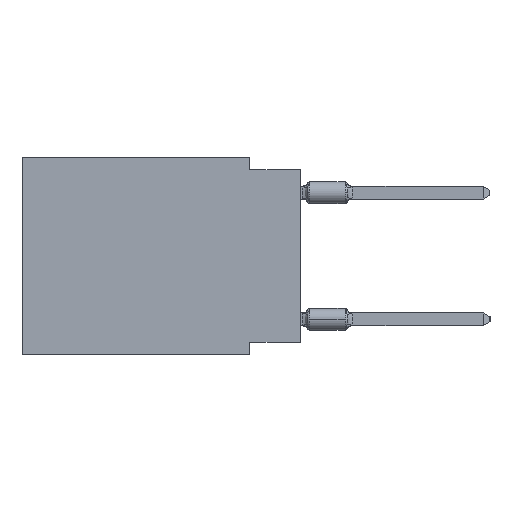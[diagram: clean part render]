
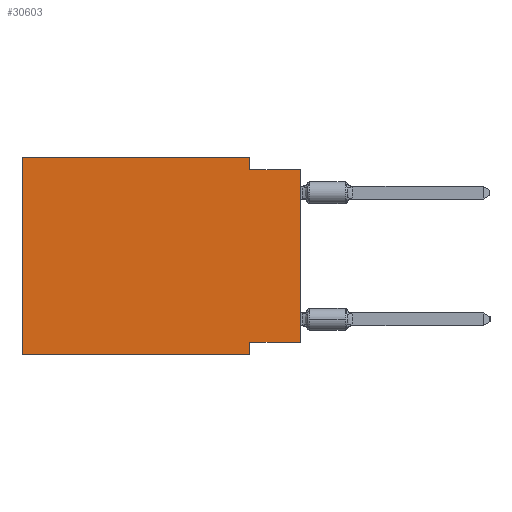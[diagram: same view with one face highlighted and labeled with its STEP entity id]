
A CAD part, left-side view. The second image highlights one B-rep face of the part: STEP entity #30603.
In plain terms, the highlighted planar face has unit normal (-1, 0, 0).
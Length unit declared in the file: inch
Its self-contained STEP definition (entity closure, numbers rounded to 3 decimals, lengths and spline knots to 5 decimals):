
#1316 = CARTESIAN_POINT ( 'NONE',  ( 0., 0.1, 0. ) ) ;
#1933 = EDGE_CURVE ( 'NONE', #29544, #7991, #47977, .T. ) ;
#4544 = DIRECTION ( 'NONE',  ( 0., 1., 0. ) ) ;
#4840 = FACE_OUTER_BOUND ( 'NONE', #44132, .T. ) ;
#5607 = VERTEX_POINT ( 'NONE', #27219 ) ;
#6581 = CARTESIAN_POINT ( 'NONE',  ( 0., 0.1, -0.365 ) ) ;
#7967 = CARTESIAN_POINT ( 'NONE',  ( 0., 0., -0.365 ) ) ;
#7991 = VERTEX_POINT ( 'NONE', #42795 ) ;
#8551 = ORIENTED_EDGE ( 'NONE', *, *, #11767, .F. ) ;
#9756 = LINE ( 'NONE', #56071, #59518 ) ;
#10496 = VERTEX_POINT ( 'NONE', #6581 ) ;
#10567 = LINE ( 'NONE', #16376, #41901 ) ;
#11022 = VERTEX_POINT ( 'NONE', #48261 ) ;
#11767 = EDGE_CURVE ( 'NONE', #47451, #29544, #20997, .T. ) ;
#12686 = CARTESIAN_POINT ( 'NONE',  ( 0., 0.55, 0. ) ) ;
#12874 = ORIENTED_EDGE ( 'NONE', *, *, #43140, .F. ) ;
#14507 = VECTOR ( 'NONE', #36011, 39.37008 ) ;
#14711 = EDGE_CURVE ( 'NONE', #5607, #11022, #17626, .T. ) ;
#16376 = CARTESIAN_POINT ( 'NONE',  ( 0., 0., -0.025 ) ) ;
#16868 = CARTESIAN_POINT ( 'NONE',  ( 0., 0.55, -0.39 ) ) ;
#17626 = LINE ( 'NONE', #45534, #57797 ) ;
#18525 = VECTOR ( 'NONE', #27995, 39.37008 ) ;
#20997 = LINE ( 'NONE', #12686, #14507 ) ;
#23380 = LINE ( 'NONE', #56791, #18525 ) ;
#23572 = DIRECTION ( 'NONE',  ( 1., 0., 0. ) ) ;
#24297 = ORIENTED_EDGE ( 'NONE', *, *, #55354, .F. ) ;
#25605 = ORIENTED_EDGE ( 'NONE', *, *, #1933, .F. ) ;
#26970 = DIRECTION ( 'NONE',  ( 0., -1., 0. ) ) ;
#27219 = CARTESIAN_POINT ( 'NONE',  ( 0., 0., -0.365 ) ) ;
#27995 = DIRECTION ( 'NONE',  ( 0., 0., 1. ) ) ;
#28317 = EDGE_CURVE ( 'NONE', #7991, #11022, #10567, .T. ) ;
#29544 = VERTEX_POINT ( 'NONE', #54392 ) ;
#29685 = CARTESIAN_POINT ( 'NONE',  ( 0., 0.55, 0. ) ) ;
#30205 = AXIS2_PLACEMENT_3D ( 'NONE', #37084, #23572, #37987 ) ;
#30603 = ADVANCED_FACE ( 'NONE', ( #4840 ), #37394, .F. ) ;
#30870 = ORIENTED_EDGE ( 'NONE', *, *, #40388, .F. ) ;
#31449 = DIRECTION ( 'NONE',  ( 0., 0., 1. ) ) ;
#32510 = EDGE_CURVE ( 'NONE', #48642, #41353, #58862, .T. ) ;
#32788 = DIRECTION ( 'NONE',  ( 0., 0., -1. ) ) ;
#34596 = ORIENTED_EDGE ( 'NONE', *, *, #32510, .T. ) ;
#36011 = DIRECTION ( 'NONE',  ( 0., -1., 0. ) ) ;
#37084 = CARTESIAN_POINT ( 'NONE',  ( 0., 0.55, 0. ) ) ;
#37394 = PLANE ( 'NONE',  #30205 ) ;
#37987 = DIRECTION ( 'NONE',  ( 0., 0., -1. ) ) ;
#38805 = DIRECTION ( 'NONE',  ( 0., -1., 0. ) ) ;
#39270 = ORIENTED_EDGE ( 'NONE', *, *, #14711, .T. ) ;
#40388 = EDGE_CURVE ( 'NONE', #10496, #41353, #9756, .T. ) ;
#40484 = CARTESIAN_POINT ( 'NONE',  ( 0., 0.1, -0.39 ) ) ;
#41353 = VERTEX_POINT ( 'NONE', #40484 ) ;
#41901 = VECTOR ( 'NONE', #38805, 39.37008 ) ;
#42795 = CARTESIAN_POINT ( 'NONE',  ( 0., 0.1, -0.025 ) ) ;
#43140 = EDGE_CURVE ( 'NONE', #48642, #47451, #23380, .T. ) ;
#44132 = EDGE_LOOP ( 'NONE', ( #39270, #59857, #25605, #8551, #12874, #34596, #30870, #24297 ) ) ;
#45534 = CARTESIAN_POINT ( 'NONE',  ( 0., 0., 0. ) ) ;
#46600 = LINE ( 'NONE', #7967, #54746 ) ;
#47451 = VERTEX_POINT ( 'NONE', #29685 ) ;
#47460 = VECTOR ( 'NONE', #51660, 39.37008 ) ;
#47977 = LINE ( 'NONE', #1316, #47460 ) ;
#48261 = CARTESIAN_POINT ( 'NONE',  ( 0., 0., -0.025 ) ) ;
#48642 = VERTEX_POINT ( 'NONE', #57262 ) ;
#51660 = DIRECTION ( 'NONE',  ( 0., 0., -1. ) ) ;
#54392 = CARTESIAN_POINT ( 'NONE',  ( 0., 0.1, 0. ) ) ;
#54746 = VECTOR ( 'NONE', #4544, 39.37008 ) ;
#55354 = EDGE_CURVE ( 'NONE', #5607, #10496, #46600, .T. ) ;
#56071 = CARTESIAN_POINT ( 'NONE',  ( 0., 0.1, -0.39 ) ) ;
#56791 = CARTESIAN_POINT ( 'NONE',  ( 0., 0.55, 0. ) ) ;
#57262 = CARTESIAN_POINT ( 'NONE',  ( 0., 0.55, -0.39 ) ) ;
#57797 = VECTOR ( 'NONE', #31449, 39.37008 ) ;
#58759 = VECTOR ( 'NONE', #26970, 39.37008 ) ;
#58862 = LINE ( 'NONE', #16868, #58759 ) ;
#59518 = VECTOR ( 'NONE', #32788, 39.37008 ) ;
#59857 = ORIENTED_EDGE ( 'NONE', *, *, #28317, .F. ) ;
